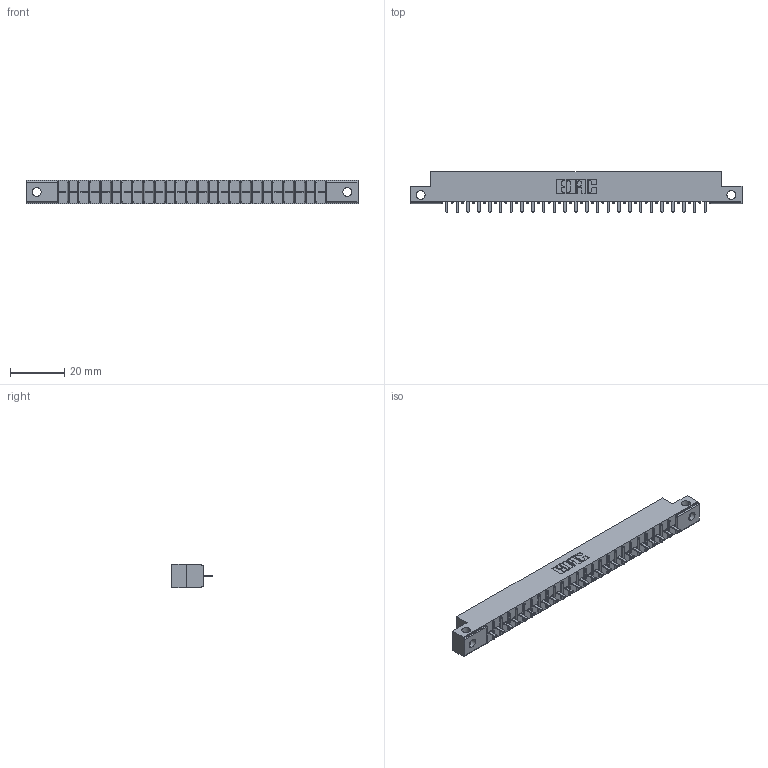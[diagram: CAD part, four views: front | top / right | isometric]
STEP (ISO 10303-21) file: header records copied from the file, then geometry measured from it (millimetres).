
FILE_DESCRIPTION (( 'STEP AP203' ), '1' );
FILE_NAME ('356-025-421-112.STEP', '2020-09-23T17:07:07', ( '' ), ( '' ), 'SwSTEP 2.0', 'SolidWorks 2020', '' );
FILE_SCHEMA (( 'CONFIG_CONTROL_DESIGN' ));
Length unit declared in the file: inch
Products named in the file (3): 356-025-421-112; 306-290-001_121; 306 Part_.128 Dia
Assembly tree (26 placements, depth 2):
  356-025-421-112
    306 Part_.128 Dia
    306-290-001_121  x25
Bounding box: 122.07 x 14.88 x 8.71 mm (x, y, z)
Volume: 8190.4 mm3; surface area: 11984.6 mm2
Topology: 26 solids, 26 shells, 1878 faces, 5277 edges, 3378 vertices
Faces by surface type: plane 1243, cylinder 535, sphere 100
Entity records: 25878 total; most frequent: CARTESIAN_POINT 4390, ORIENTED_EDGE 4306, DIRECTION 4269, EDGE_CURVE 2153, VECTOR 1659, LINE 1659, VERTEX_POINT 1362, AXIS2_PLACEMENT_3D 1305
